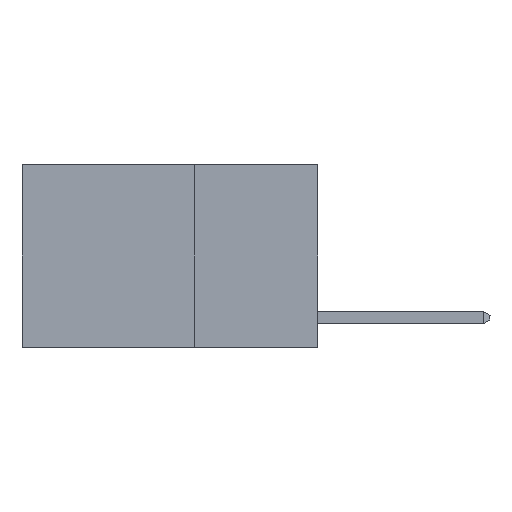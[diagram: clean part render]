
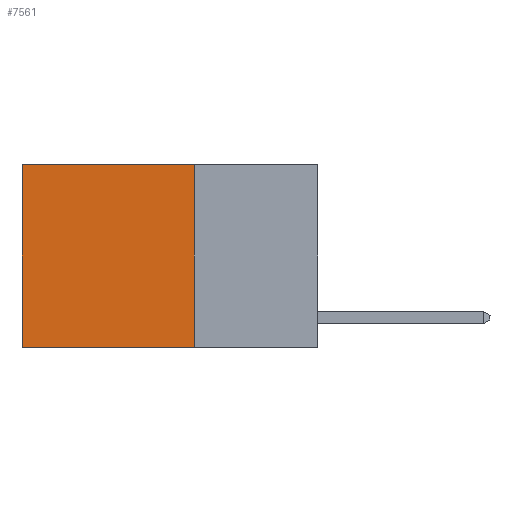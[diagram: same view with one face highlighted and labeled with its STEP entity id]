
A CAD part, left-side view. The second image highlights one B-rep face of the part: STEP entity #7561.
In plain terms, the highlighted planar face has unit normal (-1, 0, 0).
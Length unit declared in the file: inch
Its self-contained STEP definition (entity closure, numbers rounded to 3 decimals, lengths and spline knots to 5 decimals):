
#289 = VERTEX_POINT ( 'NONE', #3739 ) ;
#364 = EDGE_CURVE ( 'NONE', #11027, #289, #19070, .T. ) ;
#851 = VECTOR ( 'NONE', #18278, 39.37008 ) ;
#977 = DIRECTION ( 'NONE',  ( 0., 1., 0. ) ) ;
#2058 = VECTOR ( 'NONE', #5813, 39.37008 ) ;
#3548 = LINE ( 'NONE', #13837, #2058 ) ;
#3739 = CARTESIAN_POINT ( 'NONE',  ( 0.2625, 0.6, -0.37 ) ) ;
#4419 = DIRECTION ( 'NONE',  ( 1., 0., 0. ) ) ;
#4441 = CARTESIAN_POINT ( 'NONE',  ( 0.2625, 0.25, 0. ) ) ;
#4597 = EDGE_LOOP ( 'NONE', ( #15573, #5975, #5070, #7909 ) ) ;
#5045 = EDGE_CURVE ( 'NONE', #15148, #11027, #8156, .T. ) ;
#5070 = ORIENTED_EDGE ( 'NONE', *, *, #5045, .F. ) ;
#5329 = VECTOR ( 'NONE', #977, 39.37008 ) ;
#5430 = EDGE_CURVE ( 'NONE', #15148, #9324, #5642, .T. ) ;
#5642 = LINE ( 'NONE', #4441, #851 ) ;
#5813 = DIRECTION ( 'NONE',  ( 0., 0., -1. ) ) ;
#5975 = ORIENTED_EDGE ( 'NONE', *, *, #364, .F. ) ;
#7329 = CARTESIAN_POINT ( 'NONE',  ( 0.2625, 0.25, -0.37 ) ) ;
#7561 = ADVANCED_FACE ( 'NONE', ( #11562 ), #10807, .F. ) ;
#7769 = CARTESIAN_POINT ( 'NONE',  ( 0.2625, 0.6, 0. ) ) ;
#7909 = ORIENTED_EDGE ( 'NONE', *, *, #5430, .T. ) ;
#8131 = CARTESIAN_POINT ( 'NONE',  ( 0.2625, 0.25, 0. ) ) ;
#8156 = LINE ( 'NONE', #8131, #19139 ) ;
#9324 = VERTEX_POINT ( 'NONE', #7769 ) ;
#10807 = PLANE ( 'NONE',  #20286 ) ;
#11027 = VERTEX_POINT ( 'NONE', #7329 ) ;
#11562 = FACE_OUTER_BOUND ( 'NONE', #4597, .T. ) ;
#11638 = CARTESIAN_POINT ( 'NONE',  ( 0.2625, 0.25, 0. ) ) ;
#11765 = CARTESIAN_POINT ( 'NONE',  ( 0.2625, 0.25, 0. ) ) ;
#12308 = CARTESIAN_POINT ( 'NONE',  ( 0.2625, 0.25, -0.37 ) ) ;
#13101 = DIRECTION ( 'NONE',  ( 0., 0., -1. ) ) ;
#13837 = CARTESIAN_POINT ( 'NONE',  ( 0.2625, 0.6, 0. ) ) ;
#15148 = VERTEX_POINT ( 'NONE', #11765 ) ;
#15573 = ORIENTED_EDGE ( 'NONE', *, *, #16635, .T. ) ;
#16635 = EDGE_CURVE ( 'NONE', #9324, #289, #3548, .T. ) ;
#18278 = DIRECTION ( 'NONE',  ( 0., 1., 0. ) ) ;
#19070 = LINE ( 'NONE', #12308, #5329 ) ;
#19139 = VECTOR ( 'NONE', #13101, 39.37008 ) ;
#20109 = DIRECTION ( 'NONE',  ( 0., 0., -1. ) ) ;
#20286 = AXIS2_PLACEMENT_3D ( 'NONE', #11638, #4419, #20109 ) ;
